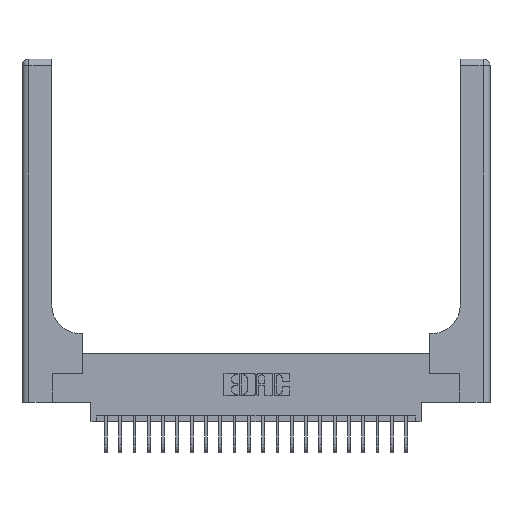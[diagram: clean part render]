
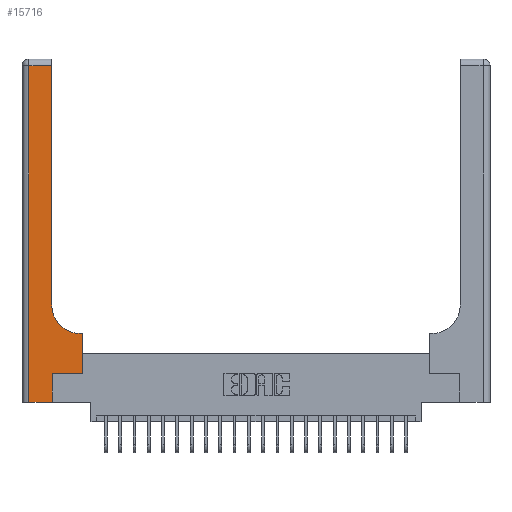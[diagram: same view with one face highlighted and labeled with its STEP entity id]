
A CAD part, top view. The second image highlights one B-rep face of the part: STEP entity #15716.
In plain terms, the highlighted planar face has unit normal (0, 0, 1).
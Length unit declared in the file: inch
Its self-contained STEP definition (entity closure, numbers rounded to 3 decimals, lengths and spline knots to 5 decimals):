
#613 = PLANE ( 'NONE',  #17091 ) ;
#860 = ORIENTED_EDGE ( 'NONE', *, *, #12732, .T. ) ;
#954 = CARTESIAN_POINT ( 'NONE',  ( 0.06, 3., 0.37 ) ) ;
#990 = VERTEX_POINT ( 'NONE', #12689 ) ;
#1217 = VERTEX_POINT ( 'NONE', #3247 ) ;
#1431 = VECTOR ( 'NONE', #15363, 39.37008 ) ;
#1463 = LINE ( 'NONE', #954, #18215 ) ;
#1540 = CARTESIAN_POINT ( 'NONE',  ( 0.51, 0.6, 0.37 ) ) ;
#1686 = CARTESIAN_POINT ( 'NONE',  ( 0., 0., 0.37 ) ) ;
#2120 = CARTESIAN_POINT ( 'NONE',  ( 0.51, 0.85, 0.37 ) ) ;
#2143 = CIRCLE ( 'NONE', #3503, 0.25 ) ;
#2336 = CARTESIAN_POINT ( 'NONE',  ( 0.06, 0., 0.37 ) ) ;
#2464 = DIRECTION ( 'NONE',  ( 0., 1., 0. ) ) ;
#3247 = CARTESIAN_POINT ( 'NONE',  ( 0.265, 0., 0.37 ) ) ;
#3503 = AXIS2_PLACEMENT_3D ( 'NONE', #2120, #13839, #3807 ) ;
#3807 = DIRECTION ( 'NONE',  ( 1., 0., 0. ) ) ;
#4041 = DIRECTION ( 'NONE',  ( 0., 0., -1. ) ) ;
#4164 = FACE_OUTER_BOUND ( 'NONE', #16747, .T. ) ;
#4208 = LINE ( 'NONE', #1686, #17017 ) ;
#4539 = VECTOR ( 'NONE', #16445, 39.37008 ) ;
#4843 = CARTESIAN_POINT ( 'NONE',  ( 0.06, 2.94, 0.37 ) ) ;
#5040 = CARTESIAN_POINT ( 'NONE',  ( 0.528, 0.6, 0.37 ) ) ;
#5250 = CARTESIAN_POINT ( 'NONE',  ( 0.265, 0., 0.37 ) ) ;
#5776 = ORIENTED_EDGE ( 'NONE', *, *, #8082, .T. ) ;
#5845 = CARTESIAN_POINT ( 'NONE',  ( 0.26, 3., 0.37 ) ) ;
#6202 = VECTOR ( 'NONE', #13837, 39.37008 ) ;
#6594 = VECTOR ( 'NONE', #15577, 39.37008 ) ;
#7010 = CARTESIAN_POINT ( 'NONE',  ( 0.265, 0.25, 0.37 ) ) ;
#7166 = CARTESIAN_POINT ( 'NONE',  ( 0.26, 0.85, 0.37 ) ) ;
#7212 = CARTESIAN_POINT ( 'NONE',  ( 0.265, 0.25, 0.37 ) ) ;
#7396 = VERTEX_POINT ( 'NONE', #1540 ) ;
#7698 = VECTOR ( 'NONE', #15423, 39.37008 ) ;
#7958 = VERTEX_POINT ( 'NONE', #5040 ) ;
#8082 = EDGE_CURVE ( 'NONE', #9662, #20821, #10325, .T. ) ;
#8252 = EDGE_CURVE ( 'NONE', #11710, #990, #11122, .T. ) ;
#8766 = CARTESIAN_POINT ( 'NONE',  ( 0.26, 0.6, 0.37 ) ) ;
#9654 = EDGE_CURVE ( 'NONE', #1217, #9662, #11065, .T. ) ;
#9662 = VERTEX_POINT ( 'NONE', #7212 ) ;
#10325 = LINE ( 'NONE', #7010, #1431 ) ;
#10336 = EDGE_CURVE ( 'NONE', #10547, #10921, #1463, .T. ) ;
#10547 = VERTEX_POINT ( 'NONE', #4843 ) ;
#10598 = ORIENTED_EDGE ( 'NONE', *, *, #8252, .T. ) ;
#10646 = LINE ( 'NONE', #8766, #6202 ) ;
#10789 = EDGE_CURVE ( 'NONE', #7958, #7396, #10646, .T. ) ;
#10921 = VERTEX_POINT ( 'NONE', #2336 ) ;
#11065 = LINE ( 'NONE', #5250, #6594 ) ;
#11122 = LINE ( 'NONE', #5845, #15580 ) ;
#11710 = VERTEX_POINT ( 'NONE', #7166 ) ;
#12689 = CARTESIAN_POINT ( 'NONE',  ( 0.26, 2.94, 0.37 ) ) ;
#12732 = EDGE_CURVE ( 'NONE', #20821, #7958, #13970, .T. ) ;
#13534 = CARTESIAN_POINT ( 'NONE',  ( 0.528, 0.25, 0.37 ) ) ;
#13718 = CARTESIAN_POINT ( 'NONE',  ( 0., 2.94, 0.37 ) ) ;
#13837 = DIRECTION ( 'NONE',  ( -1., 0., 0. ) ) ;
#13839 = DIRECTION ( 'NONE',  ( 0., 0., -1. ) ) ;
#13970 = LINE ( 'NONE', #14755, #4539 ) ;
#14391 = DIRECTION ( 'NONE',  ( 0., -1., 0. ) ) ;
#14623 = ORIENTED_EDGE ( 'NONE', *, *, #10336, .T. ) ;
#14755 = CARTESIAN_POINT ( 'NONE',  ( 0.528, 0.25, 0.37 ) ) ;
#15363 = DIRECTION ( 'NONE',  ( 1., 0., 0. ) ) ;
#15423 = DIRECTION ( 'NONE',  ( -1., 0., 0. ) ) ;
#15577 = DIRECTION ( 'NONE',  ( 0., 1., 0. ) ) ;
#15580 = VECTOR ( 'NONE', #2464, 39.37008 ) ;
#15716 = ADVANCED_FACE ( 'NONE', ( #4164 ), #613, .F. ) ;
#15746 = DIRECTION ( 'NONE',  ( -1., 0., 0. ) ) ;
#16445 = DIRECTION ( 'NONE',  ( 0., 1., 0. ) ) ;
#16545 = EDGE_CURVE ( 'NONE', #7396, #11710, #2143, .T. ) ;
#16747 = EDGE_LOOP ( 'NONE', ( #10598, #18642, #14623, #17746, #21675, #5776, #860, #19913, #20841 ) ) ;
#17017 = VECTOR ( 'NONE', #18459, 39.37008 ) ;
#17091 = AXIS2_PLACEMENT_3D ( 'NONE', #19028, #4041, #15746 ) ;
#17746 = ORIENTED_EDGE ( 'NONE', *, *, #17785, .T. ) ;
#17785 = EDGE_CURVE ( 'NONE', #10921, #1217, #4208, .T. ) ;
#18215 = VECTOR ( 'NONE', #14391, 39.37008 ) ;
#18459 = DIRECTION ( 'NONE',  ( 1., 0., 0. ) ) ;
#18642 = ORIENTED_EDGE ( 'NONE', *, *, #21417, .T. ) ;
#19028 = CARTESIAN_POINT ( 'NONE',  ( 0., 3., 0.37 ) ) ;
#19913 = ORIENTED_EDGE ( 'NONE', *, *, #10789, .T. ) ;
#20517 = LINE ( 'NONE', #13718, #7698 ) ;
#20821 = VERTEX_POINT ( 'NONE', #13534 ) ;
#20841 = ORIENTED_EDGE ( 'NONE', *, *, #16545, .T. ) ;
#21417 = EDGE_CURVE ( 'NONE', #990, #10547, #20517, .T. ) ;
#21675 = ORIENTED_EDGE ( 'NONE', *, *, #9654, .T. ) ;
